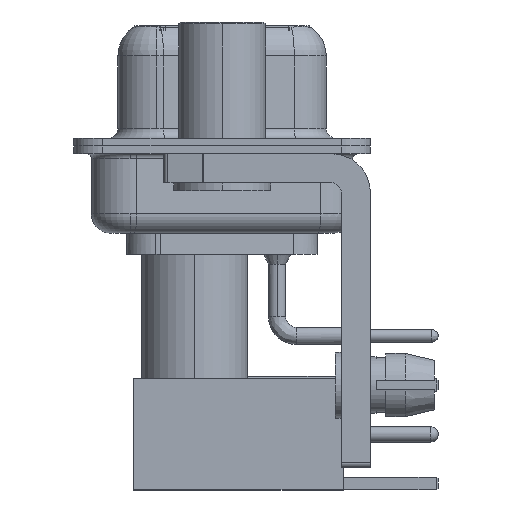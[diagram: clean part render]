
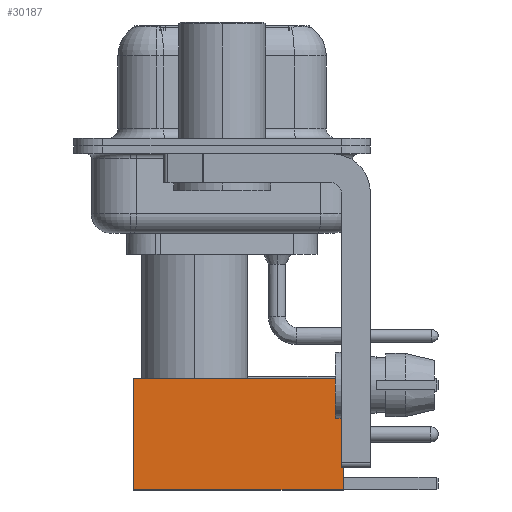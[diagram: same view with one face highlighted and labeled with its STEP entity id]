
A CAD part, left-side view. The second image highlights one B-rep face of the part: STEP entity #30187.
In plain terms, the highlighted face is planar.
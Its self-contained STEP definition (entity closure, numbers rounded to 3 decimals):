
#430 = CARTESIAN_POINT ( 'NONE',  ( 2.875, 2.875, 0. ) ) ;
#857 = DIRECTION ( 'NONE',  ( 0., 1., 0. ) ) ;
#4781 = CARTESIAN_POINT ( 'NONE',  ( 0., 2.875, 10.82 ) ) ;
#5332 = CARTESIAN_POINT ( 'NONE',  ( -2.875, 2.875, 0. ) ) ;
#6193 = ORIENTED_EDGE ( 'NONE', *, *, #15706, .F. ) ;
#8546 = EDGE_CURVE ( 'NONE', #38295, #31439, #16975, .T. ) ;
#10689 = DIRECTION ( 'NONE',  ( 0., 0., -1. ) ) ;
#10907 = DIRECTION ( 'NONE',  ( -1., 0., 0. ) ) ;
#15706 = EDGE_CURVE ( 'NONE', #19369, #38295, #33339, .T. ) ;
#16146 = VECTOR ( 'NONE', #10907, 1000. ) ;
#16975 = LINE ( 'NONE', #23447, #35053 ) ;
#17819 = ORIENTED_EDGE ( 'NONE', *, *, #8546, .F. ) ;
#19369 = VERTEX_POINT ( 'NONE', #35970 ) ;
#19888 = EDGE_LOOP ( 'NONE', ( #35600, #20635, #17819, #6193 ) ) ;
#20635 = ORIENTED_EDGE ( 'NONE', *, *, #35660, .T. ) ;
#21469 = CARTESIAN_POINT ( 'NONE',  ( -2.875, 2.875, 10.82 ) ) ;
#22605 = DIRECTION ( 'NONE',  ( 0., 0., 1. ) ) ;
#23030 = FACE_OUTER_BOUND ( 'NONE', #19888, .T. ) ;
#23447 = CARTESIAN_POINT ( 'NONE',  ( -2.875, 2.875, 0. ) ) ;
#24065 = VERTEX_POINT ( 'NONE', #36953 ) ;
#24255 = LINE ( 'NONE', #27774, #28742 ) ;
#24936 = VECTOR ( 'NONE', #33749, 1000. ) ;
#25970 = EDGE_CURVE ( 'NONE', #19369, #24065, #24255, .T. ) ;
#27774 = CARTESIAN_POINT ( 'NONE',  ( 2.875, 2.875, 0. ) ) ;
#28742 = VECTOR ( 'NONE', #36911, 1000. ) ;
#29610 = AXIS2_PLACEMENT_3D ( 'NONE', #430, #857, #22605 ) ;
#30187 = ADVANCED_FACE ( 'NONE', ( #23030 ), #35691, .T. ) ;
#31439 = VERTEX_POINT ( 'NONE', #5332 ) ;
#32995 = LINE ( 'NONE', #39836, #16146 ) ;
#33339 = LINE ( 'NONE', #4781, #24936 ) ;
#33749 = DIRECTION ( 'NONE',  ( -1., 0., 0. ) ) ;
#35053 = VECTOR ( 'NONE', #10689, 1000. ) ;
#35600 = ORIENTED_EDGE ( 'NONE', *, *, #25970, .T. ) ;
#35660 = EDGE_CURVE ( 'NONE', #24065, #31439, #32995, .T. ) ;
#35691 = PLANE ( 'NONE',  #29610 ) ;
#35970 = CARTESIAN_POINT ( 'NONE',  ( 2.875, 2.875, 10.82 ) ) ;
#36911 = DIRECTION ( 'NONE',  ( 0., 0., -1. ) ) ;
#36953 = CARTESIAN_POINT ( 'NONE',  ( 2.875, 2.875, 0. ) ) ;
#38295 = VERTEX_POINT ( 'NONE', #21469 ) ;
#39836 = CARTESIAN_POINT ( 'NONE',  ( 0., 2.875, 0. ) ) ;
